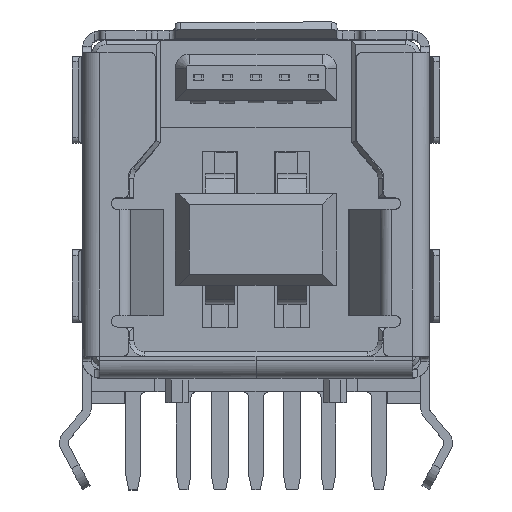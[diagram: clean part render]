
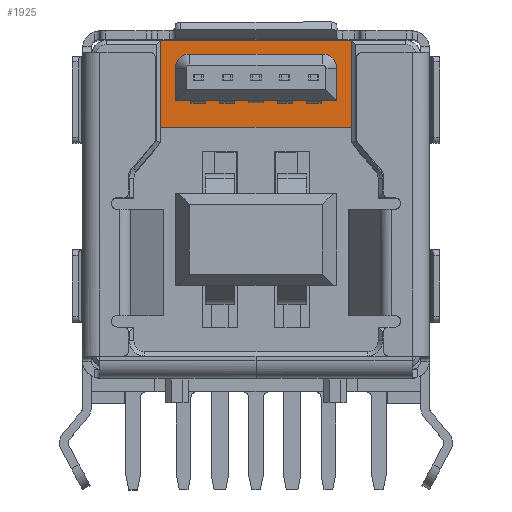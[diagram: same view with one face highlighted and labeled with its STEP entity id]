
A CAD part, top view. The second image highlights one B-rep face of the part: STEP entity #1925.
In plain terms, the highlighted planar face has unit normal (0, 0, 1).
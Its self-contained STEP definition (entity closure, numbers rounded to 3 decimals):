
#104 = VERTEX_POINT ( 'NONE', #6525 ) ;
#143 = DIRECTION ( 'NONE',  ( -1., 0., 0. ) ) ;
#398 = CARTESIAN_POINT ( 'NONE',  ( -3.295, 4.175, -8.88 ) ) ;
#889 = ORIENTED_EDGE ( 'NONE', *, *, #42579, .F. ) ;
#908 = CARTESIAN_POINT ( 'NONE',  ( 0., 2.675, -8.88 ) ) ;
#1782 = LINE ( 'NONE', #40304, #12222 ) ;
#1925 = ADVANCED_FACE ( 'NONE', ( #39438, #17977 ), #32195, .T. ) ;
#2357 = EDGE_CURVE ( 'NONE', #40674, #104, #30584, .T. ) ;
#3641 = LINE ( 'NONE', #17896, #29265 ) ;
#4297 = CARTESIAN_POINT ( 'NONE',  ( 2.295, 5.2, -8.88 ) ) ;
#4725 = EDGE_CURVE ( 'NONE', #40674, #9549, #3641, .T. ) ;
#6525 = CARTESIAN_POINT ( 'NONE',  ( 2.795, 4.7, -8.88 ) ) ;
#6646 = ORIENTED_EDGE ( 'NONE', *, *, #29301, .F. ) ;
#6755 = ORIENTED_EDGE ( 'NONE', *, *, #4725, .F. ) ;
#6948 = CARTESIAN_POINT ( 'NONE',  ( 0., 5.675, -8.88 ) ) ;
#7444 = DIRECTION ( 'NONE',  ( 0., 0., 1. ) ) ;
#7623 = LINE ( 'NONE', #43140, #33045 ) ;
#8252 = ORIENTED_EDGE ( 'NONE', *, *, #31660, .T. ) ;
#8264 = CARTESIAN_POINT ( 'NONE',  ( -2.795, 4.7, -8.88 ) ) ;
#8338 = EDGE_CURVE ( 'NONE', #13943, #25371, #21647, .T. ) ;
#8531 = DIRECTION ( 'NONE',  ( 0., 1., 0. ) ) ;
#8668 = CARTESIAN_POINT ( 'NONE',  ( 3.295, 4.175, -8.88 ) ) ;
#9549 = VERTEX_POINT ( 'NONE', #22792 ) ;
#10258 = DIRECTION ( 'NONE',  ( 1., 0., 0. ) ) ;
#10651 = DIRECTION ( 'NONE',  ( 0., 0., -1. ) ) ;
#10875 = DIRECTION ( 'NONE',  ( 0., 1., 0. ) ) ;
#11350 = CIRCLE ( 'NONE', #21044, 0.5 ) ;
#12222 = VECTOR ( 'NONE', #8531, 1000. ) ;
#13527 = VERTEX_POINT ( 'NONE', #21350 ) ;
#13681 = LINE ( 'NONE', #31652, #35917 ) ;
#13706 = ORIENTED_EDGE ( 'NONE', *, *, #15167, .F. ) ;
#13741 = VECTOR ( 'NONE', #10875, 1000. ) ;
#13943 = VERTEX_POINT ( 'NONE', #21473 ) ;
#14441 = LINE ( 'NONE', #908, #31912 ) ;
#15157 = CARTESIAN_POINT ( 'NONE',  ( -2.295, 4.7, -8.88 ) ) ;
#15167 = EDGE_CURVE ( 'NONE', #13527, #43765, #40662, .T. ) ;
#15442 = AXIS2_PLACEMENT_3D ( 'NONE', #28243, #7444, #10258 ) ;
#17067 = CARTESIAN_POINT ( 'NONE',  ( -2.795, 3.59, -8.88 ) ) ;
#17896 = CARTESIAN_POINT ( 'NONE',  ( 0., 5.2, -8.88 ) ) ;
#17977 = FACE_OUTER_BOUND ( 'NONE', #34919, .T. ) ;
#18396 = DIRECTION ( 'NONE',  ( 1., 0., 0. ) ) ;
#20297 = DIRECTION ( 'NONE',  ( 1., 0., 0. ) ) ;
#20556 = ORIENTED_EDGE ( 'NONE', *, *, #2357, .T. ) ;
#21044 = AXIS2_PLACEMENT_3D ( 'NONE', #15157, #29405, #25897 ) ;
#21350 = CARTESIAN_POINT ( 'NONE',  ( 3.295, 5.675, -8.88 ) ) ;
#21473 = CARTESIAN_POINT ( 'NONE',  ( -3.295, 2.675, -8.88 ) ) ;
#21647 = LINE ( 'NONE', #398, #13741 ) ;
#21698 = DIRECTION ( 'NONE',  ( -1., 0., 0. ) ) ;
#22792 = CARTESIAN_POINT ( 'NONE',  ( -2.295, 5.2, -8.88 ) ) ;
#23565 = CARTESIAN_POINT ( 'NONE',  ( -3.295, 5.675, -8.88 ) ) ;
#24851 = ORIENTED_EDGE ( 'NONE', *, *, #8338, .F. ) ;
#25371 = VERTEX_POINT ( 'NONE', #23565 ) ;
#25897 = DIRECTION ( 'NONE',  ( -1., 0., 0. ) ) ;
#26147 = VERTEX_POINT ( 'NONE', #8264 ) ;
#27038 = EDGE_LOOP ( 'NONE', ( #8252, #6646, #29262, #33473, #6755, #20556 ) ) ;
#27585 = AXIS2_PLACEMENT_3D ( 'NONE', #42652, #10651, #31227 ) ;
#28243 = CARTESIAN_POINT ( 'NONE',  ( -3.427, 2.615, -8.88 ) ) ;
#29262 = ORIENTED_EDGE ( 'NONE', *, *, #43518, .T. ) ;
#29265 = VECTOR ( 'NONE', #143, 1000. ) ;
#29301 = EDGE_CURVE ( 'NONE', #40074, #45519, #7623, .T. ) ;
#29405 = DIRECTION ( 'NONE',  ( 0., 0., -1. ) ) ;
#30584 = CIRCLE ( 'NONE', #27585, 0.5 ) ;
#31227 = DIRECTION ( 'NONE',  ( -1., 0., 0. ) ) ;
#31652 = CARTESIAN_POINT ( 'NONE',  ( 2.795, 4.145, -8.88 ) ) ;
#31660 = EDGE_CURVE ( 'NONE', #104, #45519, #13681, .T. ) ;
#31912 = VECTOR ( 'NONE', #21698, 1000. ) ;
#32195 = PLANE ( 'NONE',  #15442 ) ;
#33045 = VECTOR ( 'NONE', #18396, 1000. ) ;
#33473 = ORIENTED_EDGE ( 'NONE', *, *, #41460, .T. ) ;
#33881 = DIRECTION ( 'NONE',  ( 0., -1., 0. ) ) ;
#34919 = EDGE_LOOP ( 'NONE', ( #24851, #42839, #13706, #889 ) ) ;
#35917 = VECTOR ( 'NONE', #45686, 1000. ) ;
#39438 = FACE_BOUND ( 'NONE', #27038, .T. ) ;
#39490 = EDGE_CURVE ( 'NONE', #43765, #13943, #14441, .T. ) ;
#40074 = VERTEX_POINT ( 'NONE', #17067 ) ;
#40304 = CARTESIAN_POINT ( 'NONE',  ( -2.795, 4.145, -8.88 ) ) ;
#40662 = LINE ( 'NONE', #8668, #45177 ) ;
#40674 = VERTEX_POINT ( 'NONE', #4297 ) ;
#41339 = CARTESIAN_POINT ( 'NONE',  ( 3.295, 2.675, -8.88 ) ) ;
#41460 = EDGE_CURVE ( 'NONE', #26147, #9549, #11350, .T. ) ;
#42216 = LINE ( 'NONE', #6948, #43497 ) ;
#42579 = EDGE_CURVE ( 'NONE', #25371, #13527, #42216, .T. ) ;
#42652 = CARTESIAN_POINT ( 'NONE',  ( 2.295, 4.7, -8.88 ) ) ;
#42839 = ORIENTED_EDGE ( 'NONE', *, *, #39490, .F. ) ;
#43140 = CARTESIAN_POINT ( 'NONE',  ( 0., 3.59, -8.88 ) ) ;
#43497 = VECTOR ( 'NONE', #20297, 1000. ) ;
#43518 = EDGE_CURVE ( 'NONE', #40074, #26147, #1782, .T. ) ;
#43765 = VERTEX_POINT ( 'NONE', #41339 ) ;
#44645 = CARTESIAN_POINT ( 'NONE',  ( 2.795, 3.59, -8.88 ) ) ;
#45177 = VECTOR ( 'NONE', #33881, 1000. ) ;
#45519 = VERTEX_POINT ( 'NONE', #44645 ) ;
#45686 = DIRECTION ( 'NONE',  ( 0., -1., 0. ) ) ;
